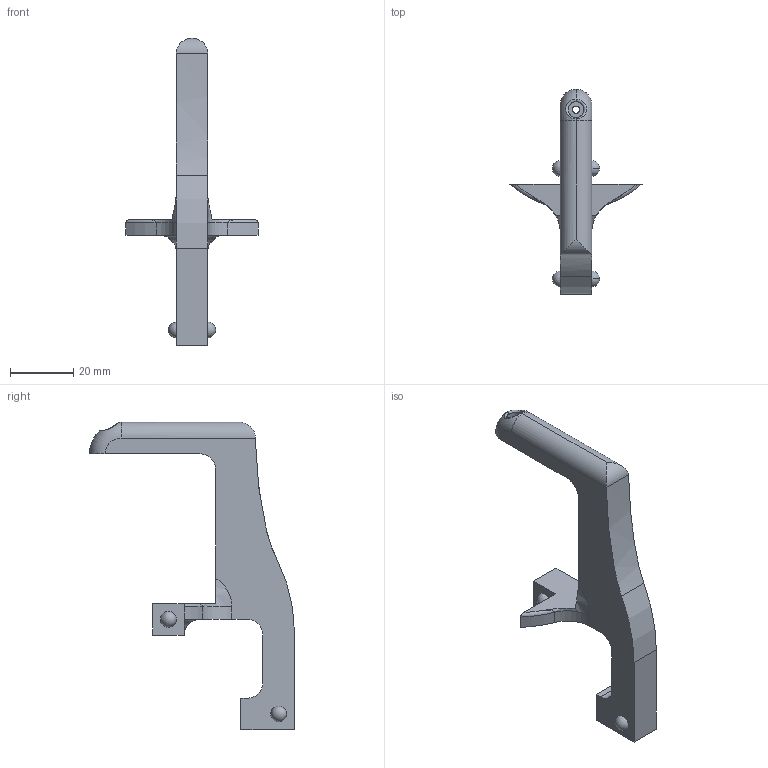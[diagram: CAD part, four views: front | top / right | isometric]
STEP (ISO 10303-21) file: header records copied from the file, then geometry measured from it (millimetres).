
FILE_DESCRIPTION (( 'STEP AP214' ), '1' );
FILE_NAME ('Trigger_Guard_Front.STEP', '2013-11-21T02:42:15', ( '' ), ( '' ), 'SwSTEP 2.0', 'SolidWorks 2013', '' );
FILE_SCHEMA (( 'AUTOMOTIVE_DESIGN' ));
Length unit declared in the file: millimetre
Products named in the file (1): Trigger_Guard_Front
Bounding box: 41.88 x 65 x 97.5 mm (x, y, z)
Volume: 20550.1 mm3; surface area: 8180.2 mm2
Topology: 1 solids, 1 shells, 51 faces, 146 edges, 93 vertices
Faces by surface type: cylinder 18, plane 18, sphere 6, bspline 5, torus 4
Entity records: 2133 total; most frequent: CARTESIAN_POINT 886, ORIENTED_EDGE 260, DIRECTION 246, EDGE_CURVE 130, AXIS2_PLACEMENT_3D 93, VERTEX_POINT 85, VECTOR 60, LINE 60
